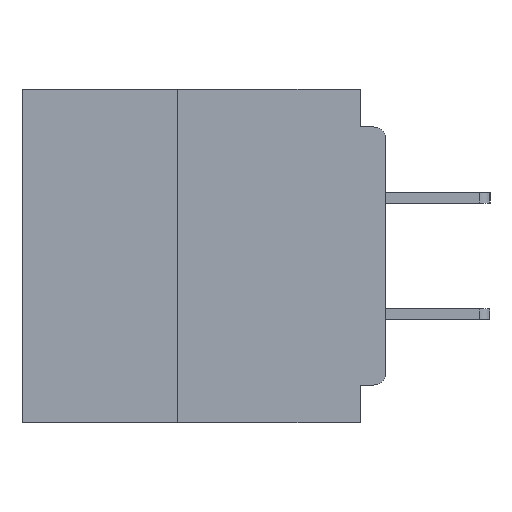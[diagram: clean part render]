
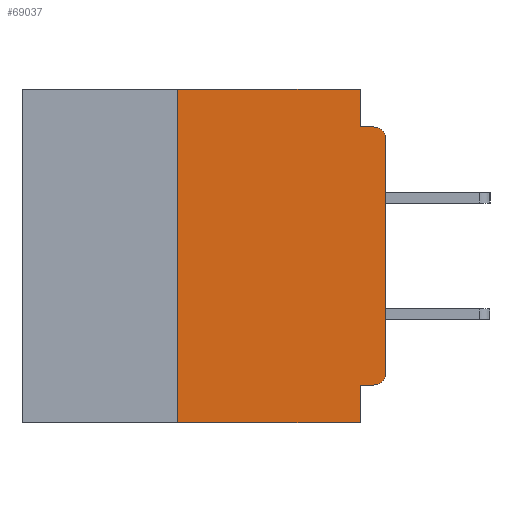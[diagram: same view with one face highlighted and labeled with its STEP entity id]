
A CAD part, left-side view. The second image highlights one B-rep face of the part: STEP entity #69037.
In plain terms, the highlighted planar face has unit normal (-1, 0, 0).
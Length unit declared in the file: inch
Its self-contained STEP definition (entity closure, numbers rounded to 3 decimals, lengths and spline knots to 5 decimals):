
#340 = CARTESIAN_POINT ( 'NONE',  ( 0., 0., -0.06 ) ) ;
#524 = AXIS2_PLACEMENT_3D ( 'NONE', #19103, #56344, #24438 ) ;
#1707 = ORIENTED_EDGE ( 'NONE', *, *, #4851, .T. ) ;
#2285 = CARTESIAN_POINT ( 'NONE',  ( 0., 0.031, -0.045 ) ) ;
#3179 = VECTOR ( 'NONE', #21721, 39.37008 ) ;
#4013 = VERTEX_POINT ( 'NONE', #9594 ) ;
#4851 = EDGE_CURVE ( 'NONE', #27224, #18090, #53134, .T. ) ;
#5532 = LINE ( 'NONE', #68794, #14727 ) ;
#7311 = DIRECTION ( 'NONE',  ( 1., 0., 0. ) ) ;
#7727 = CARTESIAN_POINT ( 'NONE',  ( 0., 0., 0. ) ) ;
#8098 = CARTESIAN_POINT ( 'NONE',  ( 0., 0.031, -0.355 ) ) ;
#8239 = VECTOR ( 'NONE', #39212, 39.37008 ) ;
#8577 = EDGE_CURVE ( 'NONE', #66857, #4013, #54230, .T. ) ;
#9181 = AXIS2_PLACEMENT_3D ( 'NONE', #23402, #7311, #34114 ) ;
#9594 = CARTESIAN_POINT ( 'NONE',  ( 0., 0.25, 0. ) ) ;
#10149 = ORIENTED_EDGE ( 'NONE', *, *, #61557, .F. ) ;
#10840 = LINE ( 'NONE', #7727, #55058 ) ;
#11178 = FACE_OUTER_BOUND ( 'NONE', #38356, .T. ) ;
#11332 = CARTESIAN_POINT ( 'NONE',  ( 0., 0.015, -0.355 ) ) ;
#11523 = CIRCLE ( 'NONE', #524, 0.015 ) ;
#11699 = VECTOR ( 'NONE', #44801, 39.37008 ) ;
#12464 = EDGE_CURVE ( 'NONE', #66857, #16195, #32879, .T. ) ;
#14727 = VECTOR ( 'NONE', #58074, 39.37008 ) ;
#14935 = LINE ( 'NONE', #55824, #57474 ) ;
#16195 = VERTEX_POINT ( 'NONE', #34671 ) ;
#18090 = VERTEX_POINT ( 'NONE', #51933 ) ;
#18288 = LINE ( 'NONE', #32371, #30745 ) ;
#19103 = CARTESIAN_POINT ( 'NONE',  ( 0., 0.015, -0.34 ) ) ;
#20176 = ORIENTED_EDGE ( 'NONE', *, *, #8577, .F. ) ;
#20960 = CARTESIAN_POINT ( 'NONE',  ( 0., 0.437, -0.4 ) ) ;
#20975 = ORIENTED_EDGE ( 'NONE', *, *, #66288, .F. ) ;
#21721 = DIRECTION ( 'NONE',  ( 0., -1., 0. ) ) ;
#23012 = ORIENTED_EDGE ( 'NONE', *, *, #27126, .F. ) ;
#23402 = CARTESIAN_POINT ( 'NONE',  ( 0., 0.437, 0. ) ) ;
#23476 = ORIENTED_EDGE ( 'NONE', *, *, #46945, .T. ) ;
#23899 = DIRECTION ( 'NONE',  ( 0., -1., 0. ) ) ;
#24438 = DIRECTION ( 'NONE',  ( 0., 0., -1. ) ) ;
#25322 = CARTESIAN_POINT ( 'NONE',  ( 0., 0.25, -0.4 ) ) ;
#25568 = EDGE_CURVE ( 'NONE', #65306, #18090, #49163, .T. ) ;
#26301 = DIRECTION ( 'NONE',  ( 0., -1., 0. ) ) ;
#27126 = EDGE_CURVE ( 'NONE', #60178, #65306, #5532, .T. ) ;
#27224 = VERTEX_POINT ( 'NONE', #340 ) ;
#28146 = CARTESIAN_POINT ( 'NONE',  ( 0., 0.015, -0.06 ) ) ;
#28759 = PLANE ( 'NONE',  #9181 ) ;
#30316 = VERTEX_POINT ( 'NONE', #44418 ) ;
#30745 = VECTOR ( 'NONE', #64305, 39.37008 ) ;
#31008 = EDGE_CURVE ( 'NONE', #30316, #27224, #10840, .T. ) ;
#31751 = EDGE_CURVE ( 'NONE', #59754, #42404, #36594, .T. ) ;
#32371 = CARTESIAN_POINT ( 'NONE',  ( 0., 0.031, -0.4 ) ) ;
#32879 = LINE ( 'NONE', #20960, #59570 ) ;
#33505 = DIRECTION ( 'NONE',  ( 0., 0., -1. ) ) ;
#33863 = CARTESIAN_POINT ( 'NONE',  ( 0., 0., -0.355 ) ) ;
#34114 = DIRECTION ( 'NONE',  ( 0., 0., -1. ) ) ;
#34671 = CARTESIAN_POINT ( 'NONE',  ( 0., 0.031, -0.4 ) ) ;
#34735 = ORIENTED_EDGE ( 'NONE', *, *, #25568, .F. ) ;
#36594 = LINE ( 'NONE', #33863, #8239 ) ;
#37334 = AXIS2_PLACEMENT_3D ( 'NONE', #28146, #65472, #33505 ) ;
#37449 = ORIENTED_EDGE ( 'NONE', *, *, #31751, .F. ) ;
#38356 = EDGE_LOOP ( 'NONE', ( #65584, #1707, #34735, #23012, #10149, #20176, #43142, #20975, #37449, #23476 ) ) ;
#39212 = DIRECTION ( 'NONE',  ( 0., 1., 0. ) ) ;
#42404 = VERTEX_POINT ( 'NONE', #8098 ) ;
#42931 = CARTESIAN_POINT ( 'NONE',  ( 0., 0., -0.045 ) ) ;
#43142 = ORIENTED_EDGE ( 'NONE', *, *, #12464, .T. ) ;
#44418 = CARTESIAN_POINT ( 'NONE',  ( 0., 0., -0.34 ) ) ;
#44801 = DIRECTION ( 'NONE',  ( 0., 0., 1. ) ) ;
#45004 = DIRECTION ( 'NONE',  ( 0., 0., 1. ) ) ;
#46684 = CARTESIAN_POINT ( 'NONE',  ( 0., 0.031, 0. ) ) ;
#46945 = EDGE_CURVE ( 'NONE', #59754, #30316, #11523, .T. ) ;
#49163 = LINE ( 'NONE', #42931, #3179 ) ;
#51933 = CARTESIAN_POINT ( 'NONE',  ( 0., 0.015, -0.045 ) ) ;
#53134 = CIRCLE ( 'NONE', #37334, 0.015 ) ;
#54230 = LINE ( 'NONE', #66036, #11699 ) ;
#55058 = VECTOR ( 'NONE', #45004, 39.37008 ) ;
#55824 = CARTESIAN_POINT ( 'NONE',  ( 0., 0.437, 0. ) ) ;
#56344 = DIRECTION ( 'NONE',  ( -1., 0., 0. ) ) ;
#57474 = VECTOR ( 'NONE', #23899, 39.37008 ) ;
#58074 = DIRECTION ( 'NONE',  ( 0., 0., -1. ) ) ;
#59570 = VECTOR ( 'NONE', #26301, 39.37008 ) ;
#59754 = VERTEX_POINT ( 'NONE', #11332 ) ;
#60178 = VERTEX_POINT ( 'NONE', #46684 ) ;
#61557 = EDGE_CURVE ( 'NONE', #4013, #60178, #14935, .T. ) ;
#64305 = DIRECTION ( 'NONE',  ( 0., 0., -1. ) ) ;
#65306 = VERTEX_POINT ( 'NONE', #2285 ) ;
#65472 = DIRECTION ( 'NONE',  ( -1., 0., 0. ) ) ;
#65584 = ORIENTED_EDGE ( 'NONE', *, *, #31008, .T. ) ;
#66036 = CARTESIAN_POINT ( 'NONE',  ( 0., 0.25, -0.4 ) ) ;
#66288 = EDGE_CURVE ( 'NONE', #42404, #16195, #18288, .T. ) ;
#66857 = VERTEX_POINT ( 'NONE', #25322 ) ;
#68794 = CARTESIAN_POINT ( 'NONE',  ( 0., 0.031, 0. ) ) ;
#69037 = ADVANCED_FACE ( 'NONE', ( #11178 ), #28759, .F. ) ;
